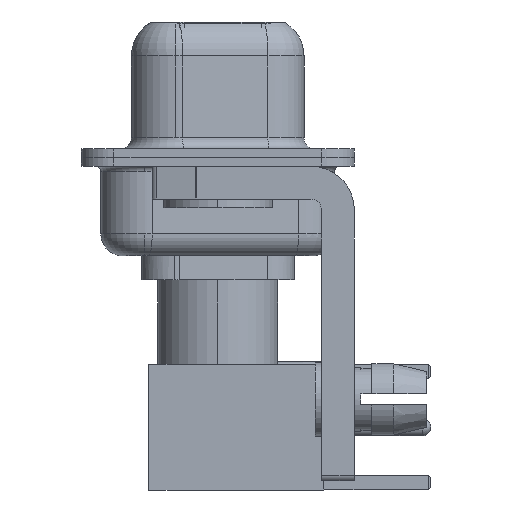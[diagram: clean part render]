
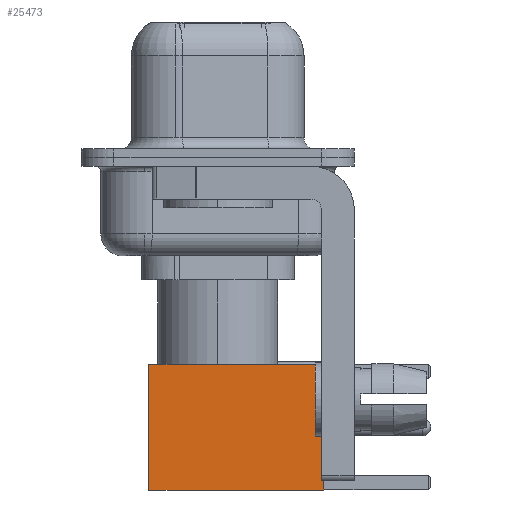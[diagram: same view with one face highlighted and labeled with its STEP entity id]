
A CAD part, left-side view. The second image highlights one B-rep face of the part: STEP entity #25473.
In plain terms, the highlighted face is planar.
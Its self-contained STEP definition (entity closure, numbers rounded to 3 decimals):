
#89 = PLANE ( 'NONE',  #13791 ) ;
#1609 = EDGE_CURVE ( 'NONE', #13901, #5384, #24572, .T. ) ;
#2126 = FACE_OUTER_BOUND ( 'NONE', #4635, .T. ) ;
#2774 = VECTOR ( 'NONE', #14821, 1000. ) ;
#3990 = ORIENTED_EDGE ( 'NONE', *, *, #14565, .F. ) ;
#4163 = DIRECTION ( 'NONE',  ( 0., 0., 1. ) ) ;
#4635 = EDGE_LOOP ( 'NONE', ( #26320, #16319, #3990, #24074 ) ) ;
#4676 = VECTOR ( 'NONE', #5645, 1000. ) ;
#5384 = VERTEX_POINT ( 'NONE', #25471 ) ;
#5645 = DIRECTION ( 'NONE',  ( -1., 0., 0. ) ) ;
#5837 = VERTEX_POINT ( 'NONE', #10604 ) ;
#6316 = LINE ( 'NONE', #14326, #13827 ) ;
#9988 = DIRECTION ( 'NONE',  ( -1., 0., 0. ) ) ;
#10604 = CARTESIAN_POINT ( 'NONE',  ( -2.875, 2.875, 0. ) ) ;
#12432 = DIRECTION ( 'NONE',  ( 0., 0., -1. ) ) ;
#12433 = CARTESIAN_POINT ( 'NONE',  ( 2.875, 2.875, 0. ) ) ;
#13791 = AXIS2_PLACEMENT_3D ( 'NONE', #12433, #22795, #4163 ) ;
#13827 = VECTOR ( 'NONE', #12432, 1000. ) ;
#13901 = VERTEX_POINT ( 'NONE', #15896 ) ;
#14326 = CARTESIAN_POINT ( 'NONE',  ( -2.875, 2.875, 0. ) ) ;
#14565 = EDGE_CURVE ( 'NONE', #5384, #5837, #6316, .T. ) ;
#14821 = DIRECTION ( 'NONE',  ( 0., 0., -1. ) ) ;
#15896 = CARTESIAN_POINT ( 'NONE',  ( 2.875, 2.875, 8. ) ) ;
#16265 = VERTEX_POINT ( 'NONE', #17451 ) ;
#16319 = ORIENTED_EDGE ( 'NONE', *, *, #25358, .T. ) ;
#17451 = CARTESIAN_POINT ( 'NONE',  ( 2.875, 2.875, 0. ) ) ;
#17514 = LINE ( 'NONE', #25820, #2774 ) ;
#18807 = VECTOR ( 'NONE', #9988, 1000. ) ;
#20337 = LINE ( 'NONE', #22393, #4676 ) ;
#22393 = CARTESIAN_POINT ( 'NONE',  ( 0., 2.875, 0. ) ) ;
#22568 = EDGE_CURVE ( 'NONE', #13901, #16265, #17514, .T. ) ;
#22795 = DIRECTION ( 'NONE',  ( 0., 1., 0. ) ) ;
#24074 = ORIENTED_EDGE ( 'NONE', *, *, #1609, .F. ) ;
#24572 = LINE ( 'NONE', #24832, #18807 ) ;
#24832 = CARTESIAN_POINT ( 'NONE',  ( 0., 2.875, 8. ) ) ;
#25358 = EDGE_CURVE ( 'NONE', #16265, #5837, #20337, .T. ) ;
#25471 = CARTESIAN_POINT ( 'NONE',  ( -2.875, 2.875, 8. ) ) ;
#25473 = ADVANCED_FACE ( 'NONE', ( #2126 ), #89, .T. ) ;
#25820 = CARTESIAN_POINT ( 'NONE',  ( 2.875, 2.875, 0. ) ) ;
#26320 = ORIENTED_EDGE ( 'NONE', *, *, #22568, .T. ) ;
